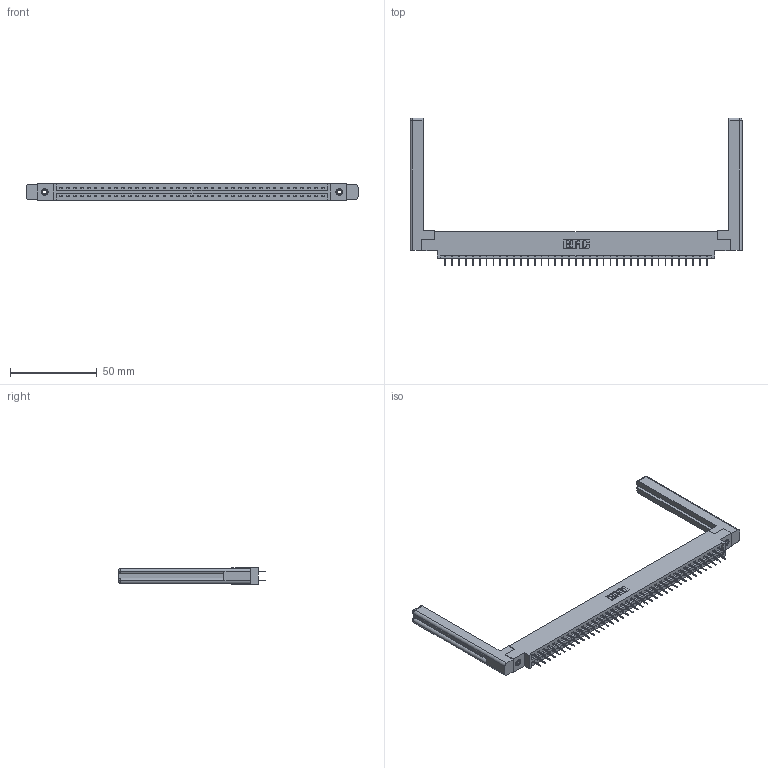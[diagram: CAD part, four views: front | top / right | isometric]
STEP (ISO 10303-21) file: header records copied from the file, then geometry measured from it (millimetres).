
FILE_DESCRIPTION (( 'STEP AP203' ), '1' );
FILE_NAME ('337-078-524-858.STEP', '2019-10-15T14:12:46', ( '' ), ( '' ), 'SwSTEP 2.0', 'SolidWorks 2016', '' );
FILE_SCHEMA (( 'CONFIG_CONTROL_DESIGN' ));
Length unit declared in the file: inch
Products named in the file (5): 337 Part_0.170 Offset - 0.156 Dia-TI; 307-220-058; 345-250-001_345-250-001-102; 337-078-524-858; 345-292-001_345-293-124
Assembly tree (83 placements, depth 2):
  337-078-524-858
    337 Part_0.170 Offset - 0.156 Dia-TI
    345-292-001_345-293-124  x78
    345-250-001_345-250-001-102  x2
    307-220-058  x2
Bounding box: 191.16 x 85.1 x 9.4 mm (x, y, z)
Volume: 27012.9 mm3; surface area: 27223.5 mm2
Topology: 83 solids, 83 shells, 4784 faces, 13547 edges, 8706 vertices
Faces by surface type: plane 3590, cylinder 1170, cone 12, torus 12
Entity records: 33466 total; most frequent: CARTESIAN_POINT 5649, ORIENTED_EDGE 5524, DIRECTION 4826, EDGE_CURVE 2762, LINE 2590, VECTOR 2590, VERTEX_POINT 1830, AXIS2_PLACEMENT_3D 1118
